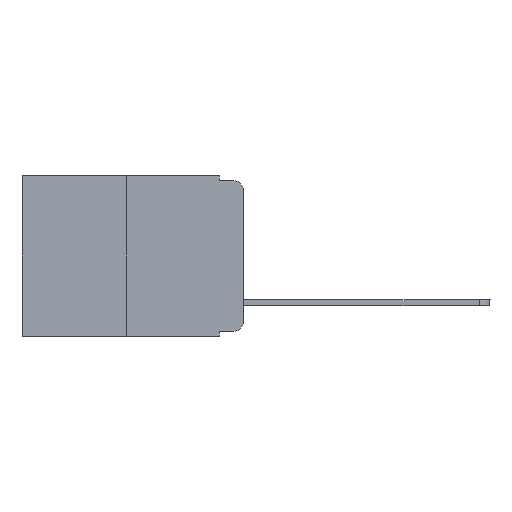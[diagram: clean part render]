
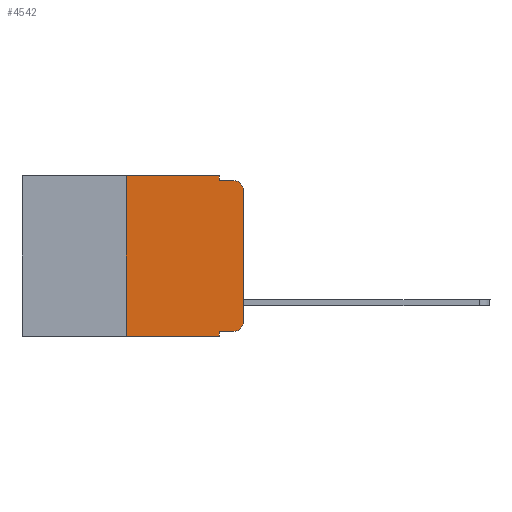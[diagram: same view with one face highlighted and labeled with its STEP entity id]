
A CAD part, left-side view. The second image highlights one B-rep face of the part: STEP entity #4542.
In plain terms, the highlighted planar face has unit normal (-1, 0, 0).
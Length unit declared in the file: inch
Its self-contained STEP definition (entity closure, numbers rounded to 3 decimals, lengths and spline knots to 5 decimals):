
#142 = LINE ( 'NONE', #22882, #20990 ) ;
#250 = DIRECTION ( 'NONE',  ( 0., -1., 0. ) ) ;
#824 = CARTESIAN_POINT ( 'NONE',  ( 0., 0.051, -0.343 ) ) ;
#1598 = EDGE_LOOP ( 'NONE', ( #22565, #25594, #13131, #7816, #12454, #18746, #17719, #13187, #25994, #8661 ) ) ;
#1733 = EDGE_CURVE ( 'NONE', #12003, #3065, #3229, .T. ) ;
#1742 = LINE ( 'NONE', #5044, #21634 ) ;
#2487 = VECTOR ( 'NONE', #14044, 39.37008 ) ;
#2932 = CARTESIAN_POINT ( 'NONE',  ( 0., 0.25, 0. ) ) ;
#3065 = VERTEX_POINT ( 'NONE', #824 ) ;
#3229 = LINE ( 'NONE', #8796, #8274 ) ;
#3398 = CARTESIAN_POINT ( 'NONE',  ( 0., 0.02, -0.333 ) ) ;
#3617 = CARTESIAN_POINT ( 'NONE',  ( 0., 0.25, -0.343 ) ) ;
#3634 = VERTEX_POINT ( 'NONE', #2932 ) ;
#3716 = VECTOR ( 'NONE', #5003, 39.37008 ) ;
#3897 = EDGE_CURVE ( 'NONE', #4893, #3634, #10041, .T. ) ;
#4067 = CARTESIAN_POINT ( 'NONE',  ( 0., 0.473, 0. ) ) ;
#4542 = ADVANCED_FACE ( 'NONE', ( #26114 ), #10135, .F. ) ;
#4617 = EDGE_CURVE ( 'NONE', #10017, #22523, #5268, .T. ) ;
#4857 = DIRECTION ( 'NONE',  ( 0., 0., -1. ) ) ;
#4893 = VERTEX_POINT ( 'NONE', #3617 ) ;
#5003 = DIRECTION ( 'NONE',  ( 0., 0., -1. ) ) ;
#5044 = CARTESIAN_POINT ( 'NONE',  ( 0., 0.473, -0.343 ) ) ;
#5268 = LINE ( 'NONE', #12280, #25817 ) ;
#5680 = EDGE_CURVE ( 'NONE', #3634, #22916, #142, .T. ) ;
#6102 = AXIS2_PLACEMENT_3D ( 'NONE', #4067, #16130, #14225 ) ;
#6357 = EDGE_CURVE ( 'NONE', #4893, #3065, #1742, .T. ) ;
#6966 = CIRCLE ( 'NONE', #13096, 0.02 ) ;
#7031 = CARTESIAN_POINT ( 'NONE',  ( 0., 0., -0.03 ) ) ;
#7215 = DIRECTION ( 'NONE',  ( 0., -1., 0. ) ) ;
#7323 = LINE ( 'NONE', #11925, #16803 ) ;
#7788 = EDGE_CURVE ( 'NONE', #23065, #8764, #7323, .T. ) ;
#7816 = ORIENTED_EDGE ( 'NONE', *, *, #20761, .F. ) ;
#8274 = VECTOR ( 'NONE', #22652, 39.37008 ) ;
#8385 = EDGE_CURVE ( 'NONE', #8764, #22523, #6966, .T. ) ;
#8661 = ORIENTED_EDGE ( 'NONE', *, *, #10537, .T. ) ;
#8662 = DIRECTION ( 'NONE',  ( 0., 0., -1. ) ) ;
#8764 = VERTEX_POINT ( 'NONE', #7031 ) ;
#8796 = CARTESIAN_POINT ( 'NONE',  ( 0., 0.051, 0. ) ) ;
#8954 = CARTESIAN_POINT ( 'NONE',  ( 0., 0.051, 0. ) ) ;
#9106 = VECTOR ( 'NONE', #11917, 39.37008 ) ;
#10017 = VERTEX_POINT ( 'NONE', #21233 ) ;
#10041 = LINE ( 'NONE', #23795, #9106 ) ;
#10135 = PLANE ( 'NONE',  #6102 ) ;
#10146 = VERTEX_POINT ( 'NONE', #3398 ) ;
#10537 = EDGE_CURVE ( 'NONE', #10146, #23065, #16939, .T. ) ;
#10827 = DIRECTION ( 'NONE',  ( 0., -1., 0. ) ) ;
#11917 = DIRECTION ( 'NONE',  ( 0., 0., 1. ) ) ;
#11925 = CARTESIAN_POINT ( 'NONE',  ( 0., 0., 0. ) ) ;
#12003 = VERTEX_POINT ( 'NONE', #13818 ) ;
#12280 = CARTESIAN_POINT ( 'NONE',  ( 0., 0.051, -0.01 ) ) ;
#12454 = ORIENTED_EDGE ( 'NONE', *, *, #5680, .F. ) ;
#12772 = EDGE_CURVE ( 'NONE', #12003, #10146, #16363, .T. ) ;
#13096 = AXIS2_PLACEMENT_3D ( 'NONE', #16636, #13911, #4857 ) ;
#13131 = ORIENTED_EDGE ( 'NONE', *, *, #4617, .F. ) ;
#13187 = ORIENTED_EDGE ( 'NONE', *, *, #1733, .F. ) ;
#13818 = CARTESIAN_POINT ( 'NONE',  ( 0., 0.051, -0.333 ) ) ;
#13911 = DIRECTION ( 'NONE',  ( -1., 0., 0. ) ) ;
#14044 = DIRECTION ( 'NONE',  ( 0., -1., 0. ) ) ;
#14225 = DIRECTION ( 'NONE',  ( 0., 0., -1. ) ) ;
#14891 = CARTESIAN_POINT ( 'NONE',  ( 0., 0.051, 0. ) ) ;
#15050 = DIRECTION ( 'NONE',  ( -1., 0., 0. ) ) ;
#16130 = DIRECTION ( 'NONE',  ( 1., 0., 0. ) ) ;
#16363 = LINE ( 'NONE', #18165, #2487 ) ;
#16636 = CARTESIAN_POINT ( 'NONE',  ( 0., 0.02, -0.03 ) ) ;
#16803 = VECTOR ( 'NONE', #26016, 39.37008 ) ;
#16939 = CIRCLE ( 'NONE', #21741, 0.02 ) ;
#17719 = ORIENTED_EDGE ( 'NONE', *, *, #6357, .T. ) ;
#18165 = CARTESIAN_POINT ( 'NONE',  ( 0., 0.051, -0.333 ) ) ;
#18746 = ORIENTED_EDGE ( 'NONE', *, *, #3897, .F. ) ;
#19163 = LINE ( 'NONE', #8954, #3716 ) ;
#20761 = EDGE_CURVE ( 'NONE', #22916, #10017, #19163, .T. ) ;
#20990 = VECTOR ( 'NONE', #10827, 39.37008 ) ;
#21029 = CARTESIAN_POINT ( 'NONE',  ( 0., 0.02, -0.313 ) ) ;
#21233 = CARTESIAN_POINT ( 'NONE',  ( 0., 0.051, -0.01 ) ) ;
#21290 = CARTESIAN_POINT ( 'NONE',  ( 0., 0., -0.313 ) ) ;
#21634 = VECTOR ( 'NONE', #7215, 39.37008 ) ;
#21741 = AXIS2_PLACEMENT_3D ( 'NONE', #21029, #15050, #8662 ) ;
#21773 = CARTESIAN_POINT ( 'NONE',  ( 0., 0.02, -0.01 ) ) ;
#22523 = VERTEX_POINT ( 'NONE', #21773 ) ;
#22565 = ORIENTED_EDGE ( 'NONE', *, *, #7788, .T. ) ;
#22652 = DIRECTION ( 'NONE',  ( 0., 0., -1. ) ) ;
#22882 = CARTESIAN_POINT ( 'NONE',  ( 0., 0.473, 0. ) ) ;
#22916 = VERTEX_POINT ( 'NONE', #14891 ) ;
#23065 = VERTEX_POINT ( 'NONE', #21290 ) ;
#23795 = CARTESIAN_POINT ( 'NONE',  ( 0., 0.25, 0. ) ) ;
#25594 = ORIENTED_EDGE ( 'NONE', *, *, #8385, .T. ) ;
#25817 = VECTOR ( 'NONE', #250, 39.37008 ) ;
#25994 = ORIENTED_EDGE ( 'NONE', *, *, #12772, .T. ) ;
#26016 = DIRECTION ( 'NONE',  ( 0., 0., 1. ) ) ;
#26114 = FACE_OUTER_BOUND ( 'NONE', #1598, .T. ) ;
